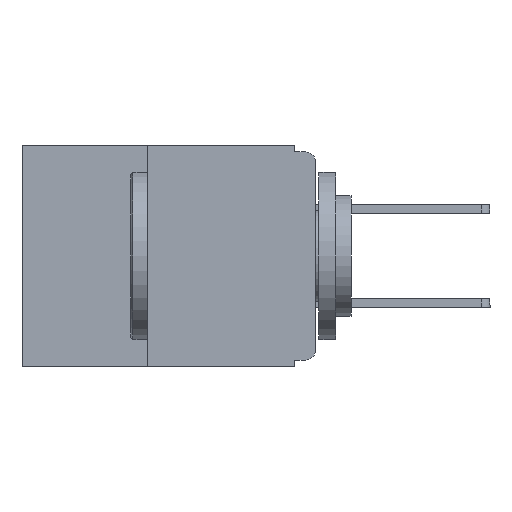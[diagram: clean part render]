
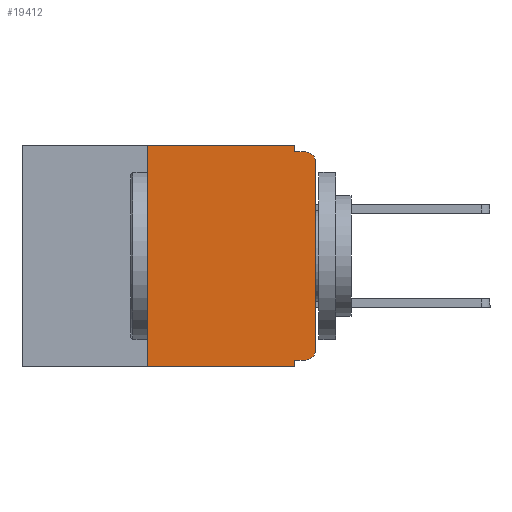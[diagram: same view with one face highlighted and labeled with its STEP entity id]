
A CAD part, left-side view. The second image highlights one B-rep face of the part: STEP entity #19412.
In plain terms, the highlighted planar face has unit normal (-1, 0, 0).
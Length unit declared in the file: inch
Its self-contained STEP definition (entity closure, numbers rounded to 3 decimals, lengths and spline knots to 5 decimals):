
#22 = FACE_OUTER_BOUND ( 'NONE', #153, .T. ) ;
#153 = EDGE_LOOP ( 'NONE', ( #7385, #4510, #8892, #9264, #7923, #4099, #12370, #1630, #10191, #2333 ) ) ;
#154 = LINE ( 'NONE', #5501, #7955 ) ;
#627 = VERTEX_POINT ( 'NONE', #11866 ) ;
#1630 = ORIENTED_EDGE ( 'NONE', *, *, #2304, .F. ) ;
#1770 = EDGE_CURVE ( 'NONE', #7592, #7349, #18890, .T. ) ;
#1953 = VERTEX_POINT ( 'NONE', #4612 ) ;
#2274 = EDGE_CURVE ( 'NONE', #10536, #1953, #7694, .T. ) ;
#2304 = EDGE_CURVE ( 'NONE', #14872, #2721, #16141, .T. ) ;
#2333 = ORIENTED_EDGE ( 'NONE', *, *, #2274, .T. ) ;
#2366 = CARTESIAN_POINT ( 'NONE',  ( 0., 0., -0.025 ) ) ;
#2407 = EDGE_CURVE ( 'NONE', #16935, #7592, #5779, .T. ) ;
#2721 = VERTEX_POINT ( 'NONE', #16602 ) ;
#3454 = VECTOR ( 'NONE', #12023, 39.37008 ) ;
#3784 = CARTESIAN_POINT ( 'NONE',  ( 0., 0.015, -0.32 ) ) ;
#4099 = ORIENTED_EDGE ( 'NONE', *, *, #19358, .F. ) ;
#4271 = VERTEX_POINT ( 'NONE', #2366 ) ;
#4510 = ORIENTED_EDGE ( 'NONE', *, *, #8430, .T. ) ;
#4612 = CARTESIAN_POINT ( 'NONE',  ( 0., 0., -0.305 ) ) ;
#4942 = PLANE ( 'NONE',  #11979 ) ;
#4979 = CARTESIAN_POINT ( 'NONE',  ( 0., 0.031, 0. ) ) ;
#5012 = CARTESIAN_POINT ( 'NONE',  ( 0., 0.437, 0. ) ) ;
#5501 = CARTESIAN_POINT ( 'NONE',  ( 0., 0., -0.32 ) ) ;
#5565 = CARTESIAN_POINT ( 'NONE',  ( 0., 0.031, -0.01 ) ) ;
#5779 = LINE ( 'NONE', #4979, #17273 ) ;
#6268 = CARTESIAN_POINT ( 'NONE',  ( 0., 0., -0.01 ) ) ;
#6561 = DIRECTION ( 'NONE',  ( 0., 0., -1. ) ) ;
#6630 = VECTOR ( 'NONE', #7263, 39.37008 ) ;
#6812 = DIRECTION ( 'NONE',  ( 0., -1., 0. ) ) ;
#6880 = VERTEX_POINT ( 'NONE', #15127 ) ;
#7142 = CARTESIAN_POINT ( 'NONE',  ( 0., 0.031, -0.33 ) ) ;
#7263 = DIRECTION ( 'NONE',  ( 0., 0., 1. ) ) ;
#7349 = VERTEX_POINT ( 'NONE', #9234 ) ;
#7385 = ORIENTED_EDGE ( 'NONE', *, *, #19080, .T. ) ;
#7578 = VECTOR ( 'NONE', #9254, 39.37008 ) ;
#7592 = VERTEX_POINT ( 'NONE', #5565 ) ;
#7694 = CIRCLE ( 'NONE', #17676, 0.015 ) ;
#7923 = ORIENTED_EDGE ( 'NONE', *, *, #11019, .F. ) ;
#7955 = VECTOR ( 'NONE', #14629, 39.37008 ) ;
#8430 = EDGE_CURVE ( 'NONE', #4271, #7349, #16125, .T. ) ;
#8724 = DIRECTION ( 'NONE',  ( 0., 0., -1. ) ) ;
#8892 = ORIENTED_EDGE ( 'NONE', *, *, #1770, .F. ) ;
#8959 = DIRECTION ( 'NONE',  ( -1., 0., 0. ) ) ;
#8978 = CARTESIAN_POINT ( 'NONE',  ( 0., 0.437, -0.33 ) ) ;
#8990 = CARTESIAN_POINT ( 'NONE',  ( 0., 0.015, -0.025 ) ) ;
#9234 = CARTESIAN_POINT ( 'NONE',  ( 0., 0.015, -0.01 ) ) ;
#9254 = DIRECTION ( 'NONE',  ( 0., -1., 0. ) ) ;
#9264 = ORIENTED_EDGE ( 'NONE', *, *, #2407, .F. ) ;
#9291 = DIRECTION ( 'NONE',  ( 0., 0., -1. ) ) ;
#9402 = DIRECTION ( 'NONE',  ( -1., 0., 0. ) ) ;
#9462 = DIRECTION ( 'NONE',  ( 0., 0., 1. ) ) ;
#9572 = CARTESIAN_POINT ( 'NONE',  ( 0., 0.031, 0. ) ) ;
#10191 = ORIENTED_EDGE ( 'NONE', *, *, #13854, .F. ) ;
#10397 = CARTESIAN_POINT ( 'NONE',  ( 0., 0.437, 0. ) ) ;
#10532 = CARTESIAN_POINT ( 'NONE',  ( 0., 0.015, -0.305 ) ) ;
#10536 = VERTEX_POINT ( 'NONE', #3784 ) ;
#10712 = LINE ( 'NONE', #13319, #6630 ) ;
#11019 = EDGE_CURVE ( 'NONE', #6880, #16935, #12619, .T. ) ;
#11049 = EDGE_CURVE ( 'NONE', #627, #2721, #11171, .T. ) ;
#11171 = LINE ( 'NONE', #8978, #7578 ) ;
#11866 = CARTESIAN_POINT ( 'NONE',  ( 0., 0.25, -0.33 ) ) ;
#11979 = AXIS2_PLACEMENT_3D ( 'NONE', #5012, #15581, #6561 ) ;
#12023 = DIRECTION ( 'NONE',  ( 0., -1., 0. ) ) ;
#12370 = ORIENTED_EDGE ( 'NONE', *, *, #11049, .T. ) ;
#12541 = CARTESIAN_POINT ( 'NONE',  ( 0., 0.25, -0.33 ) ) ;
#12619 = LINE ( 'NONE', #10397, #3454 ) ;
#12830 = AXIS2_PLACEMENT_3D ( 'NONE', #8990, #8959, #8724 ) ;
#13319 = CARTESIAN_POINT ( 'NONE',  ( 0., 0., 0. ) ) ;
#13854 = EDGE_CURVE ( 'NONE', #10536, #14872, #154, .T. ) ;
#14629 = DIRECTION ( 'NONE',  ( 0., 1., 0. ) ) ;
#14872 = VERTEX_POINT ( 'NONE', #17670 ) ;
#15040 = VECTOR ( 'NONE', #6812, 39.37008 ) ;
#15127 = CARTESIAN_POINT ( 'NONE',  ( 0., 0.25, 0. ) ) ;
#15226 = VECTOR ( 'NONE', #9291, 39.37008 ) ;
#15343 = DIRECTION ( 'NONE',  ( 0., 0., -1. ) ) ;
#15581 = DIRECTION ( 'NONE',  ( 1., 0., 0. ) ) ;
#16125 = CIRCLE ( 'NONE', #12830, 0.015 ) ;
#16141 = LINE ( 'NONE', #7142, #15226 ) ;
#16602 = CARTESIAN_POINT ( 'NONE',  ( 0., 0.031, -0.33 ) ) ;
#16745 = VECTOR ( 'NONE', #9462, 39.37008 ) ;
#16935 = VERTEX_POINT ( 'NONE', #9572 ) ;
#17273 = VECTOR ( 'NONE', #15343, 39.37008 ) ;
#17650 = LINE ( 'NONE', #12541, #16745 ) ;
#17670 = CARTESIAN_POINT ( 'NONE',  ( 0., 0.031, -0.32 ) ) ;
#17676 = AXIS2_PLACEMENT_3D ( 'NONE', #10532, #9402, #18920 ) ;
#18890 = LINE ( 'NONE', #6268, #15040 ) ;
#18920 = DIRECTION ( 'NONE',  ( 0., 0., -1. ) ) ;
#19080 = EDGE_CURVE ( 'NONE', #1953, #4271, #10712, .T. ) ;
#19358 = EDGE_CURVE ( 'NONE', #627, #6880, #17650, .T. ) ;
#19412 = ADVANCED_FACE ( 'NONE', ( #22 ), #4942, .F. ) ;
